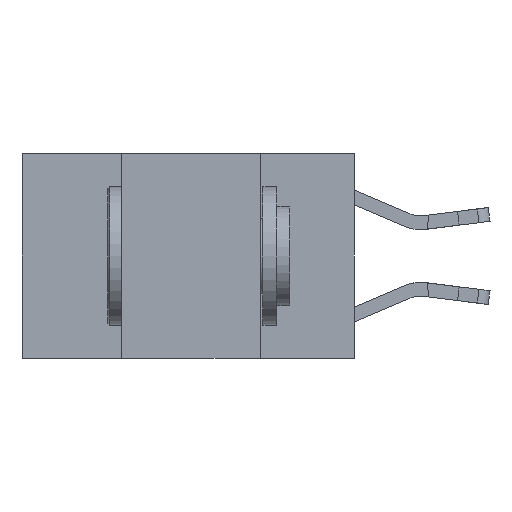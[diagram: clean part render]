
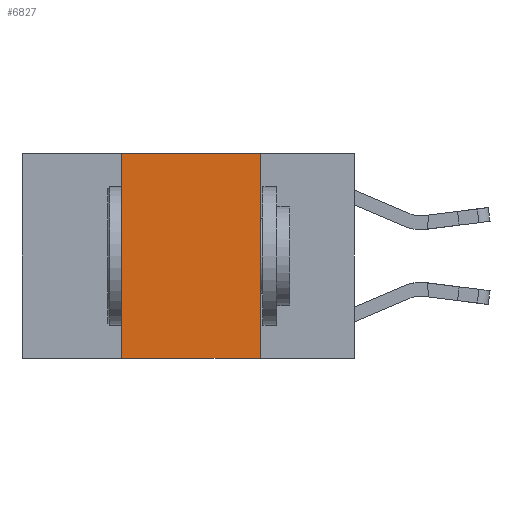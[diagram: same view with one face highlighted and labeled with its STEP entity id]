
A CAD part, left-side view. The second image highlights one B-rep face of the part: STEP entity #6827.
In plain terms, the highlighted planar face has unit normal (-1, 0, 0).
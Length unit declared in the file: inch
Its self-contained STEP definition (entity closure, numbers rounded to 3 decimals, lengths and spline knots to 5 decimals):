
#1242 = FACE_OUTER_BOUND ( 'NONE', #7684, .T. ) ;
#1616 = VECTOR ( 'NONE', #10751, 39.37008 ) ;
#2144 = EDGE_CURVE ( 'NONE', #9235, #6138, #8884, .T. ) ;
#2162 = DIRECTION ( 'NONE',  ( 0., 0., -1. ) ) ;
#2479 = CARTESIAN_POINT ( 'NONE',  ( 0., 0.6, 0. ) ) ;
#3407 = DIRECTION ( 'NONE',  ( 0., 0., -1. ) ) ;
#3417 = CARTESIAN_POINT ( 'NONE',  ( 0., 0.6, 0. ) ) ;
#3965 = VERTEX_POINT ( 'NONE', #8457 ) ;
#4529 = VECTOR ( 'NONE', #12981, 39.37008 ) ;
#4530 = CARTESIAN_POINT ( 'NONE',  ( 0., 0.17, 0. ) ) ;
#5079 = CARTESIAN_POINT ( 'NONE',  ( 0., 0.17, -0.37 ) ) ;
#5655 = CARTESIAN_POINT ( 'NONE',  ( 0., 0.42, 0. ) ) ;
#6138 = VERTEX_POINT ( 'NONE', #5655 ) ;
#6325 = ORIENTED_EDGE ( 'NONE', *, *, #2144, .F. ) ;
#6326 = ORIENTED_EDGE ( 'NONE', *, *, #7321, .F. ) ;
#6827 = ADVANCED_FACE ( 'NONE', ( #1242 ), #13220, .F. ) ;
#6842 = LINE ( 'NONE', #8857, #8435 ) ;
#7312 = DIRECTION ( 'NONE',  ( 1., 0., 0. ) ) ;
#7321 = EDGE_CURVE ( 'NONE', #3965, #12257, #10656, .T. ) ;
#7405 = EDGE_CURVE ( 'NONE', #9235, #12257, #6842, .T. ) ;
#7684 = EDGE_LOOP ( 'NONE', ( #6326, #11523, #6325, #9362 ) ) ;
#8435 = VECTOR ( 'NONE', #11178, 39.37008 ) ;
#8457 = CARTESIAN_POINT ( 'NONE',  ( 0., 0.17, 0. ) ) ;
#8857 = CARTESIAN_POINT ( 'NONE',  ( 0., 0.6, -0.37 ) ) ;
#8884 = LINE ( 'NONE', #12441, #4529 ) ;
#9235 = VERTEX_POINT ( 'NONE', #15483 ) ;
#9362 = ORIENTED_EDGE ( 'NONE', *, *, #7405, .T. ) ;
#10515 = LINE ( 'NONE', #3417, #1616 ) ;
#10656 = LINE ( 'NONE', #4530, #12158 ) ;
#10751 = DIRECTION ( 'NONE',  ( 0., -1., 0. ) ) ;
#11136 = EDGE_CURVE ( 'NONE', #6138, #3965, #10515, .T. ) ;
#11178 = DIRECTION ( 'NONE',  ( 0., -1., 0. ) ) ;
#11523 = ORIENTED_EDGE ( 'NONE', *, *, #11136, .F. ) ;
#12158 = VECTOR ( 'NONE', #3407, 39.37008 ) ;
#12257 = VERTEX_POINT ( 'NONE', #5079 ) ;
#12441 = CARTESIAN_POINT ( 'NONE',  ( 0., 0.42, 0. ) ) ;
#12981 = DIRECTION ( 'NONE',  ( 0., 0., 1. ) ) ;
#13220 = PLANE ( 'NONE',  #13992 ) ;
#13992 = AXIS2_PLACEMENT_3D ( 'NONE', #2479, #7312, #2162 ) ;
#15483 = CARTESIAN_POINT ( 'NONE',  ( 0., 0.42, -0.37 ) ) ;
